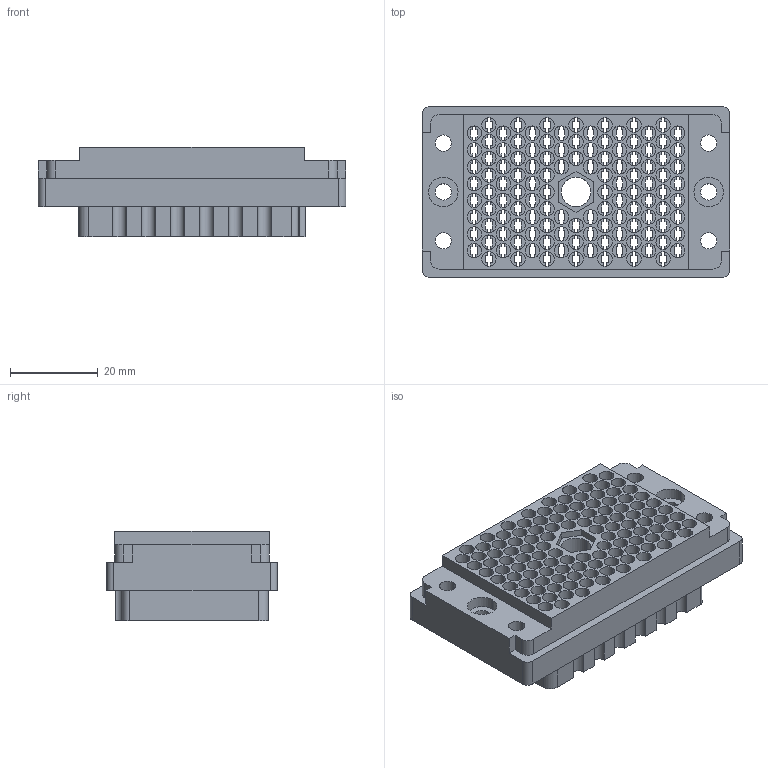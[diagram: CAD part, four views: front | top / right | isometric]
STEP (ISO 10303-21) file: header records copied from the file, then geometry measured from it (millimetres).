
FILE_DESCRIPTION (( 'STEP AP203' ), '1' );
FILE_NAME ('516-120-000-200.STEP', '2020-03-06T23:28:48', ( '' ), ( '' ), 'SwSTEP 2.0', 'SolidWorks 2016', '' );
FILE_SCHEMA (( 'CONFIG_CONTROL_DESIGN' ));
Length unit declared in the file: inch
Products named in the file (2): 516-120-000-200; 516 Part Receptacle_120
Assembly tree (1 placements, depth 2):
  516-120-000-200
    516 Part Receptacle_120
Bounding box: 69.85 x 38.73 x 20.27 mm (x, y, z)
Volume: 24521 mm3; surface area: 37577.4 mm2
Topology: 1 solids, 1 shells, 2486 faces, 7400 edges, 4932 vertices
Faces by surface type: plane 1791, cylinder 693, cone 2
Entity records: 84166 total; most frequent: CARTESIAN_POINT 14822, ORIENTED_EDGE 14800, DIRECTION 14246, EDGE_CURVE 7400, LINE 5534, VECTOR 5534, VERTEX_POINT 4932, AXIS2_PLACEMENT_3D 4356
